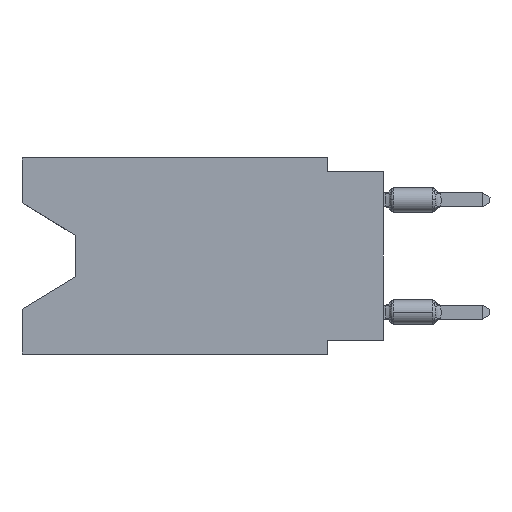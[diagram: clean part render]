
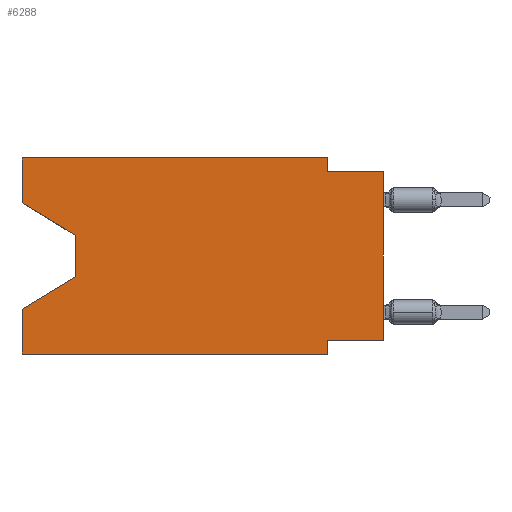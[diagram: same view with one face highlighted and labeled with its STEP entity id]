
A CAD part, left-side view. The second image highlights one B-rep face of the part: STEP entity #6288.
In plain terms, the highlighted planar face has unit normal (-1, 0, 0).
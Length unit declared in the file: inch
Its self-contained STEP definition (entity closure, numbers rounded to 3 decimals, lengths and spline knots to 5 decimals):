
#168 = ORIENTED_EDGE ( 'NONE', *, *, #13304, .T. ) ;
#365 = VERTEX_POINT ( 'NONE', #15233 ) ;
#718 = ORIENTED_EDGE ( 'NONE', *, *, #2685, .F. ) ;
#785 = ORIENTED_EDGE ( 'NONE', *, *, #2162, .F. ) ;
#935 = VECTOR ( 'NONE', #7990, 39.37008 ) ;
#1025 = CARTESIAN_POINT ( 'NONE',  ( 0., 0., -0.025 ) ) ;
#1152 = VECTOR ( 'NONE', #7260, 39.37008 ) ;
#1240 = EDGE_CURVE ( 'NONE', #5810, #8488, #11048, .T. ) ;
#1275 = CARTESIAN_POINT ( 'NONE',  ( 0., 0.1, -0.35 ) ) ;
#1306 = CARTESIAN_POINT ( 'NONE',  ( 0., 0.645, -0.08025 ) ) ;
#1600 = VECTOR ( 'NONE', #14261, 39.37008 ) ;
#1763 = VERTEX_POINT ( 'NONE', #12605 ) ;
#1857 = VECTOR ( 'NONE', #2142, 39.37008 ) ;
#2142 = DIRECTION ( 'NONE',  ( 0., -1., 0. ) ) ;
#2150 = CARTESIAN_POINT ( 'NONE',  ( 0., 0.55, -0.212 ) ) ;
#2162 = EDGE_CURVE ( 'NONE', #3783, #365, #8418, .T. ) ;
#2305 = CARTESIAN_POINT ( 'NONE',  ( 0., 0.645, -0.26975 ) ) ;
#2442 = DIRECTION ( 'NONE',  ( 0., 0., -1. ) ) ;
#2612 = EDGE_CURVE ( 'NONE', #10903, #5881, #13832, .T. ) ;
#2685 = EDGE_CURVE ( 'NONE', #10903, #3783, #6799, .T. ) ;
#2965 = DIRECTION ( 'NONE',  ( 0., -1., 0. ) ) ;
#3243 = LINE ( 'NONE', #1025, #1600 ) ;
#3419 = VECTOR ( 'NONE', #10921, 39.37008 ) ;
#3475 = DIRECTION ( 'NONE',  ( 0., 0., 1. ) ) ;
#3783 = VERTEX_POINT ( 'NONE', #7384 ) ;
#4105 = EDGE_CURVE ( 'NONE', #13839, #12079, #15506, .T. ) ;
#4302 = CARTESIAN_POINT ( 'NONE',  ( 0., 0., -0.325 ) ) ;
#4736 = LINE ( 'NONE', #10620, #5347 ) ;
#4894 = DIRECTION ( 'NONE',  ( 0., 0., 1. ) ) ;
#4897 = EDGE_CURVE ( 'NONE', #13995, #13839, #10545, .T. ) ;
#4921 = EDGE_CURVE ( 'NONE', #12079, #5881, #3243, .T. ) ;
#5347 = VECTOR ( 'NONE', #4894, 39.37008 ) ;
#5722 = CARTESIAN_POINT ( 'NONE',  ( 0., 0., 0. ) ) ;
#5810 = VERTEX_POINT ( 'NONE', #14225 ) ;
#5835 = LINE ( 'NONE', #2150, #10114 ) ;
#5881 = VERTEX_POINT ( 'NONE', #10902 ) ;
#6119 = VECTOR ( 'NONE', #2965, 39.37008 ) ;
#6288 = ADVANCED_FACE ( 'NONE', ( #9966 ), #14858, .F. ) ;
#6606 = LINE ( 'NONE', #13066, #7808 ) ;
#6722 = VERTEX_POINT ( 'NONE', #14915 ) ;
#6756 = CARTESIAN_POINT ( 'NONE',  ( 0., 0.645, 0. ) ) ;
#6799 = LINE ( 'NONE', #4302, #12248 ) ;
#6924 = DIRECTION ( 'NONE',  ( 0., 0.855, -0.519 ) ) ;
#7068 = ORIENTED_EDGE ( 'NONE', *, *, #4897, .F. ) ;
#7260 = DIRECTION ( 'NONE',  ( 0., -0.855, -0.519 ) ) ;
#7384 = CARTESIAN_POINT ( 'NONE',  ( 0., 0.1, -0.325 ) ) ;
#7391 = EDGE_CURVE ( 'NONE', #5810, #13995, #4736, .T. ) ;
#7506 = DIRECTION ( 'NONE',  ( 1., 0., 0. ) ) ;
#7808 = VECTOR ( 'NONE', #13784, 39.37008 ) ;
#7948 = EDGE_CURVE ( 'NONE', #8488, #6722, #6606, .T. ) ;
#7990 = DIRECTION ( 'NONE',  ( 0., 0., 1. ) ) ;
#8025 = ORIENTED_EDGE ( 'NONE', *, *, #4105, .F. ) ;
#8418 = LINE ( 'NONE', #1275, #3419 ) ;
#8439 = ORIENTED_EDGE ( 'NONE', *, *, #14989, .F. ) ;
#8488 = VERTEX_POINT ( 'NONE', #15136 ) ;
#8635 = CARTESIAN_POINT ( 'NONE',  ( 0., 0.1, -0.025 ) ) ;
#8831 = LINE ( 'NONE', #12636, #6119 ) ;
#9165 = DIRECTION ( 'NONE',  ( 0., 1., 0. ) ) ;
#9277 = ORIENTED_EDGE ( 'NONE', *, *, #7391, .F. ) ;
#9431 = LINE ( 'NONE', #14258, #15449 ) ;
#9498 = ORIENTED_EDGE ( 'NONE', *, *, #1240, .T. ) ;
#9585 = AXIS2_PLACEMENT_3D ( 'NONE', #13521, #7506, #12328 ) ;
#9966 = FACE_OUTER_BOUND ( 'NONE', #13867, .T. ) ;
#10083 = EDGE_CURVE ( 'NONE', #1763, #365, #8831, .T. ) ;
#10114 = VECTOR ( 'NONE', #6924, 39.37008 ) ;
#10256 = ORIENTED_EDGE ( 'NONE', *, *, #10083, .T. ) ;
#10545 = LINE ( 'NONE', #6756, #1857 ) ;
#10620 = CARTESIAN_POINT ( 'NONE',  ( 0., 0.645, 0. ) ) ;
#10902 = CARTESIAN_POINT ( 'NONE',  ( 0., 0., -0.025 ) ) ;
#10903 = VERTEX_POINT ( 'NONE', #15034 ) ;
#10921 = DIRECTION ( 'NONE',  ( 0., 0., -1. ) ) ;
#11048 = LINE ( 'NONE', #1306, #1152 ) ;
#12079 = VERTEX_POINT ( 'NONE', #8635 ) ;
#12248 = VECTOR ( 'NONE', #9165, 39.37008 ) ;
#12328 = DIRECTION ( 'NONE',  ( 0., 0., -1. ) ) ;
#12605 = CARTESIAN_POINT ( 'NONE',  ( 0., 0.645, -0.35 ) ) ;
#12636 = CARTESIAN_POINT ( 'NONE',  ( 0., 0.645, -0.35 ) ) ;
#12789 = ORIENTED_EDGE ( 'NONE', *, *, #7948, .T. ) ;
#13066 = CARTESIAN_POINT ( 'NONE',  ( 0., 0.55, -0.138 ) ) ;
#13131 = ORIENTED_EDGE ( 'NONE', *, *, #2612, .T. ) ;
#13244 = VERTEX_POINT ( 'NONE', #2305 ) ;
#13304 = EDGE_CURVE ( 'NONE', #6722, #13244, #5835, .T. ) ;
#13447 = CARTESIAN_POINT ( 'NONE',  ( 0., 0.1, 0. ) ) ;
#13521 = CARTESIAN_POINT ( 'NONE',  ( 0., 0.645, 0. ) ) ;
#13784 = DIRECTION ( 'NONE',  ( 0., 0., -1. ) ) ;
#13832 = LINE ( 'NONE', #5722, #935 ) ;
#13839 = VERTEX_POINT ( 'NONE', #13447 ) ;
#13867 = EDGE_LOOP ( 'NONE', ( #9498, #12789, #168, #8439, #10256, #785, #718, #13131, #14980, #8025, #7068, #9277 ) ) ;
#13995 = VERTEX_POINT ( 'NONE', #15016 ) ;
#14225 = CARTESIAN_POINT ( 'NONE',  ( 0., 0.645, -0.08025 ) ) ;
#14258 = CARTESIAN_POINT ( 'NONE',  ( 0., 0.645, 0. ) ) ;
#14261 = DIRECTION ( 'NONE',  ( 0., -1., 0. ) ) ;
#14388 = CARTESIAN_POINT ( 'NONE',  ( 0., 0.1, 0. ) ) ;
#14578 = VECTOR ( 'NONE', #2442, 39.37008 ) ;
#14858 = PLANE ( 'NONE',  #9585 ) ;
#14915 = CARTESIAN_POINT ( 'NONE',  ( 0., 0.55, -0.212 ) ) ;
#14980 = ORIENTED_EDGE ( 'NONE', *, *, #4921, .F. ) ;
#14989 = EDGE_CURVE ( 'NONE', #1763, #13244, #9431, .T. ) ;
#15016 = CARTESIAN_POINT ( 'NONE',  ( 0., 0.645, 0. ) ) ;
#15034 = CARTESIAN_POINT ( 'NONE',  ( 0., 0., -0.325 ) ) ;
#15136 = CARTESIAN_POINT ( 'NONE',  ( 0., 0.55, -0.138 ) ) ;
#15233 = CARTESIAN_POINT ( 'NONE',  ( 0., 0.1, -0.35 ) ) ;
#15449 = VECTOR ( 'NONE', #3475, 39.37008 ) ;
#15506 = LINE ( 'NONE', #14388, #14578 ) ;
